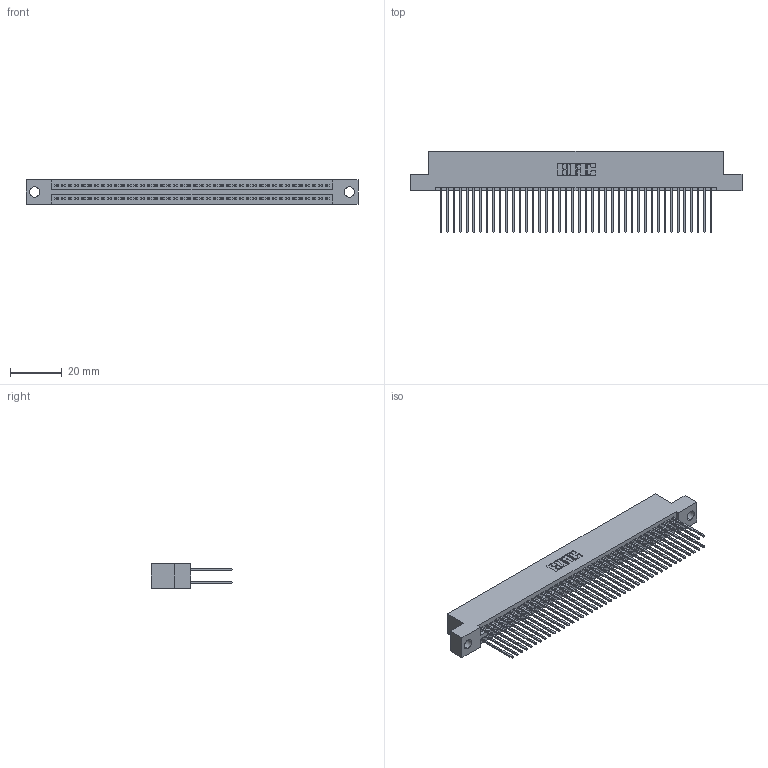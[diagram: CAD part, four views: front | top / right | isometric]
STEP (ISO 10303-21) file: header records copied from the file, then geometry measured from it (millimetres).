
FILE_DESCRIPTION (( 'STEP AP203' ), '1' );
FILE_NAME ('395-084-542-204.STEP', '2021-06-17T08:20:43', ( '' ), ( '' ), 'SwSTEP 2.0', 'SolidWorks 2020', '' );
FILE_SCHEMA (( 'CONFIG_CONTROL_DESIGN' ));
Length unit declared in the file: inch
Products named in the file (3): 395-084-542-204; 345 Part_Flush Mounting Lugs - 0.156 Dia-TI; 345-292-001_345-293-142
Assembly tree (85 placements, depth 2):
  395-084-542-204
    345 Part_Flush Mounting Lugs - 0.156 Dia-TI
    345-292-001_345-293-142  x84
Bounding box: 127.89 x 31.29 x 9.4 mm (x, y, z)
Volume: 12708.9 mm3; surface area: 20467.4 mm2
Topology: 85 solids, 85 shells, 4340 faces, 12893 edges, 8482 vertices
Faces by surface type: plane 2866, cylinder 1474
Entity records: 33391 total; most frequent: CARTESIAN_POINT 5602, ORIENTED_EDGE 5534, DIRECTION 4939, EDGE_CURVE 2767, LINE 2467, VECTOR 2467, VERTEX_POINT 1842, AXIS2_PLACEMENT_3D 1236
